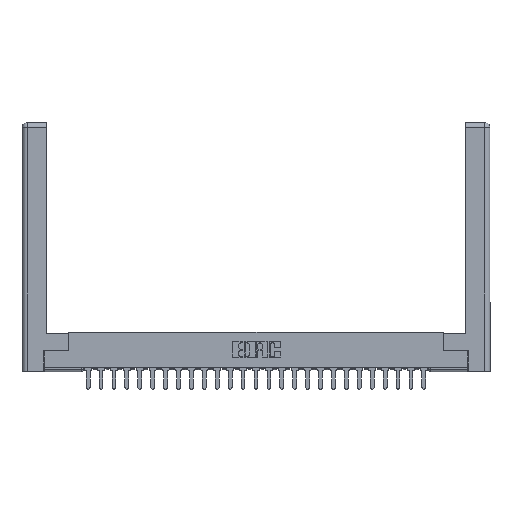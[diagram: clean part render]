
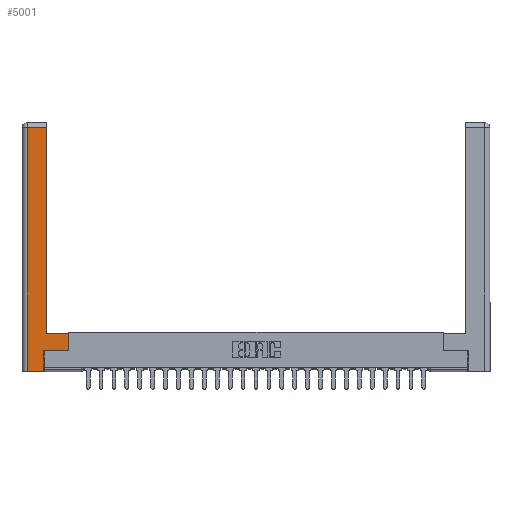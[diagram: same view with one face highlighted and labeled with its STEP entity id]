
A CAD part, top view. The second image highlights one B-rep face of the part: STEP entity #5001.
In plain terms, the highlighted planar face has unit normal (0, 0, 1).
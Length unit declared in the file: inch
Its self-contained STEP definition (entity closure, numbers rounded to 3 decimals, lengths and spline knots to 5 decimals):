
#10 = CARTESIAN_POINT ( 'NONE',  ( 0.265, 0.245, 0. ) ) ;
#338 = CARTESIAN_POINT ( 'NONE',  ( 0.0615, 0., 0. ) ) ;
#609 = CARTESIAN_POINT ( 'NONE',  ( 0.265, 0., 0. ) ) ;
#803 = LINE ( 'NONE', #24450, #10466 ) ;
#876 = FACE_OUTER_BOUND ( 'NONE', #24251, .T. ) ;
#1659 = ORIENTED_EDGE ( 'NONE', *, *, #18892, .T. ) ;
#1831 = LINE ( 'NONE', #26259, #4858 ) ;
#2599 = ORIENTED_EDGE ( 'NONE', *, *, #7295, .T. ) ;
#2795 = CARTESIAN_POINT ( 'NONE',  ( 0.295, 2.94, 0. ) ) ;
#3210 = CARTESIAN_POINT ( 'NONE',  ( 0.265, 0.245, 0. ) ) ;
#3416 = VECTOR ( 'NONE', #6862, 39.37008 ) ;
#3504 = ORIENTED_EDGE ( 'NONE', *, *, #20049, .T. ) ;
#3715 = LINE ( 'NONE', #19288, #6065 ) ;
#3897 = CARTESIAN_POINT ( 'NONE',  ( 0.565, 0.245, 0. ) ) ;
#4651 = DIRECTION ( 'NONE',  ( -1., 0., 0. ) ) ;
#4858 = VECTOR ( 'NONE', #9024, 39.37008 ) ;
#4910 = LINE ( 'NONE', #5807, #23490 ) ;
#5001 = ADVANCED_FACE ( 'NONE', ( #876 ), #11122, .F. ) ;
#5417 = DIRECTION ( 'NONE',  ( 1., 0., 0. ) ) ;
#5807 = CARTESIAN_POINT ( 'NONE',  ( 0.0615, 2.94, 0. ) ) ;
#6065 = VECTOR ( 'NONE', #23576, 39.37008 ) ;
#6179 = ORIENTED_EDGE ( 'NONE', *, *, #9012, .T. ) ;
#6393 = CARTESIAN_POINT ( 'NONE',  ( 0.565, 0.45, 0. ) ) ;
#6862 = DIRECTION ( 'NONE',  ( 0., 1., 0. ) ) ;
#7295 = EDGE_CURVE ( 'NONE', #21467, #21415, #7825, .T. ) ;
#7399 = CARTESIAN_POINT ( 'NONE',  ( 0.565, 0.45, 0. ) ) ;
#7825 = LINE ( 'NONE', #8938, #26085 ) ;
#8151 = ORIENTED_EDGE ( 'NONE', *, *, #13284, .T. ) ;
#8412 = LINE ( 'NONE', #6393, #15030 ) ;
#8938 = CARTESIAN_POINT ( 'NONE',  ( 0.295, 0.45, 0. ) ) ;
#9012 = EDGE_CURVE ( 'NONE', #13760, #17029, #3715, .T. ) ;
#9024 = DIRECTION ( 'NONE',  ( 0., 1., 0. ) ) ;
#10466 = VECTOR ( 'NONE', #5417, 39.37008 ) ;
#10916 = VERTEX_POINT ( 'NONE', #2795 ) ;
#11122 = PLANE ( 'NONE',  #22277 ) ;
#11211 = ORIENTED_EDGE ( 'NONE', *, *, #20844, .T. ) ;
#11297 = CARTESIAN_POINT ( 'NONE',  ( 0.295, 0.45, 0. ) ) ;
#12404 = EDGE_CURVE ( 'NONE', #17029, #14921, #22184, .T. ) ;
#13229 = CARTESIAN_POINT ( 'NONE',  ( 0., 0., 0. ) ) ;
#13284 = EDGE_CURVE ( 'NONE', #10916, #13760, #4910, .T. ) ;
#13318 = DIRECTION ( 'NONE',  ( -1., 0., 0. ) ) ;
#13760 = VERTEX_POINT ( 'NONE', #25334 ) ;
#14031 = EDGE_CURVE ( 'NONE', #21415, #10916, #1831, .T. ) ;
#14604 = CARTESIAN_POINT ( 'NONE',  ( 0.265, 0., 0. ) ) ;
#14921 = VERTEX_POINT ( 'NONE', #14604 ) ;
#15030 = VECTOR ( 'NONE', #25314, 39.37008 ) ;
#15564 = DIRECTION ( 'NONE',  ( 1., 0., 0. ) ) ;
#16345 = DIRECTION ( 'NONE',  ( -1., 0., 0. ) ) ;
#16487 = VECTOR ( 'NONE', #15564, 39.37008 ) ;
#17029 = VERTEX_POINT ( 'NONE', #338 ) ;
#18892 = EDGE_CURVE ( 'NONE', #25753, #19206, #803, .T. ) ;
#19206 = VERTEX_POINT ( 'NONE', #3897 ) ;
#19232 = ORIENTED_EDGE ( 'NONE', *, *, #14031, .T. ) ;
#19288 = CARTESIAN_POINT ( 'NONE',  ( 0.0615, 0., 0. ) ) ;
#19877 = ORIENTED_EDGE ( 'NONE', *, *, #12404, .T. ) ;
#20049 = EDGE_CURVE ( 'NONE', #14921, #25753, #27387, .T. ) ;
#20844 = EDGE_CURVE ( 'NONE', #19206, #21467, #8412, .T. ) ;
#21415 = VERTEX_POINT ( 'NONE', #11297 ) ;
#21467 = VERTEX_POINT ( 'NONE', #7399 ) ;
#22184 = LINE ( 'NONE', #609, #16487 ) ;
#22277 = AXIS2_PLACEMENT_3D ( 'NONE', #13229, #26051, #13318 ) ;
#23490 = VECTOR ( 'NONE', #16345, 39.37008 ) ;
#23576 = DIRECTION ( 'NONE',  ( 0., -1., 0. ) ) ;
#24251 = EDGE_LOOP ( 'NONE', ( #19232, #8151, #6179, #19877, #3504, #1659, #11211, #2599 ) ) ;
#24450 = CARTESIAN_POINT ( 'NONE',  ( 0.565, 0.245, 0. ) ) ;
#25314 = DIRECTION ( 'NONE',  ( 0., 1., 0. ) ) ;
#25334 = CARTESIAN_POINT ( 'NONE',  ( 0.0615, 2.94, 0. ) ) ;
#25753 = VERTEX_POINT ( 'NONE', #3210 ) ;
#26051 = DIRECTION ( 'NONE',  ( 0., 0., -1. ) ) ;
#26085 = VECTOR ( 'NONE', #4651, 39.37008 ) ;
#26259 = CARTESIAN_POINT ( 'NONE',  ( 0.295, 3., 0. ) ) ;
#27387 = LINE ( 'NONE', #10, #3416 ) ;
